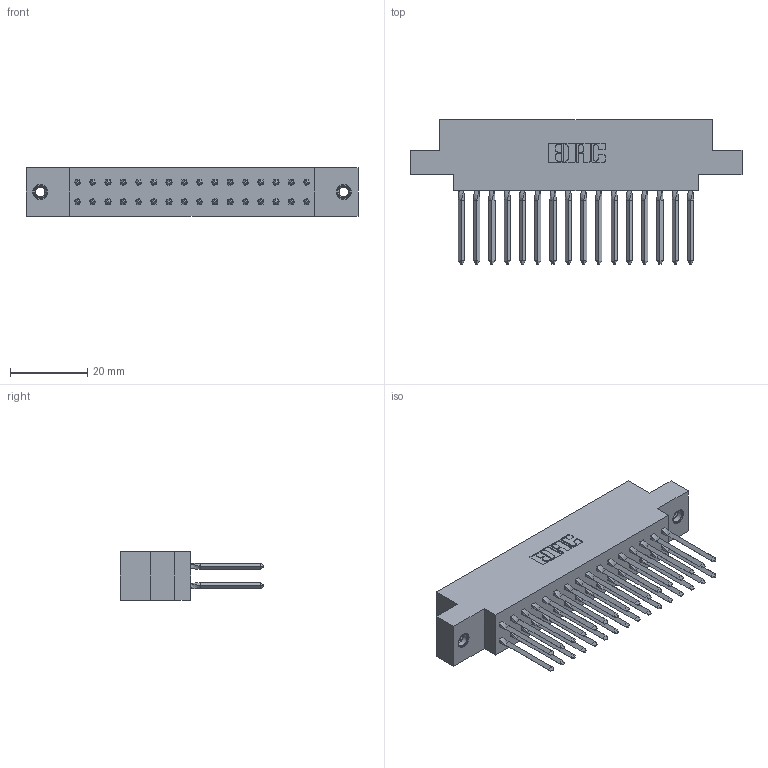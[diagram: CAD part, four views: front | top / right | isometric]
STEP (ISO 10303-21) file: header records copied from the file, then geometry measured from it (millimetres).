
FILE_DESCRIPTION (( 'STEP AP203' ), '1' );
FILE_NAME ('317-032-542-807.STEP', '2020-02-27T21:15:23', ( '' ), ( '' ), 'SwSTEP 2.0', 'SolidWorks 2016', '' );
FILE_SCHEMA (( 'CONFIG_CONTROL_DESIGN' ));
Length unit declared in the file: inch
Products named in the file (4): 317 Part_.156 Dia - TI; 317-290-003_542; 317-032-542-807; 345-250-001_345-250-005-103
Assembly tree (35 placements, depth 2):
  317-032-542-807
    317 Part_.156 Dia - TI
    317-290-003_542  x32
    345-250-001_345-250-005-103  x2
Bounding box: 86.11 x 37.34 x 12.7 mm (x, y, z)
Volume: 13264.4 mm3; surface area: 17647.4 mm2
Topology: 35 solids, 35 shells, 1986 faces, 5531 edges, 3530 vertices
Faces by surface type: plane 1562, cylinder 280, bspline 128, cone 12, torus 4
Entity records: 26958 total; most frequent: CARTESIAN_POINT 4920, ORIENTED_EDGE 4576, DIRECTION 3934, EDGE_CURVE 2288, LINE 2098, VECTOR 2098, VERTEX_POINT 1516, AXIS2_PLACEMENT_3D 918
